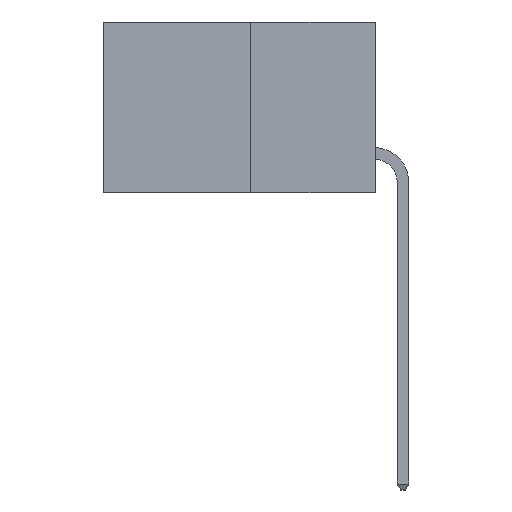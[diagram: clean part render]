
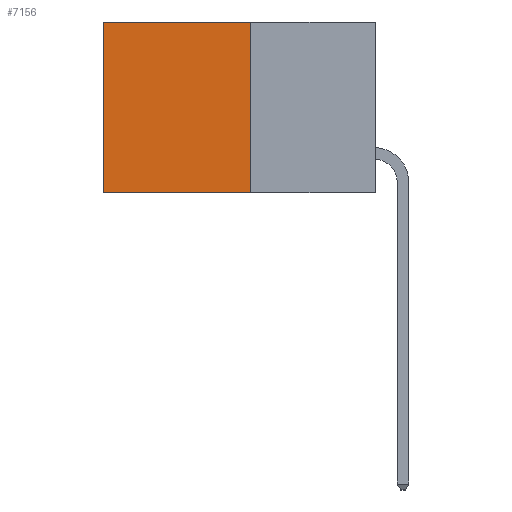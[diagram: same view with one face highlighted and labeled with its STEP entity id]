
A CAD part, left-side view. The second image highlights one B-rep face of the part: STEP entity #7156.
In plain terms, the highlighted planar face has unit normal (-1, 0, 0).
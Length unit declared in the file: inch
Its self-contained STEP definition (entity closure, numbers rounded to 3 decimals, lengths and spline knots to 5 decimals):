
#215 = DIRECTION ( 'NONE',  ( 0., 0., -1. ) ) ;
#286 = VECTOR ( 'NONE', #12590, 39.37008 ) ;
#1157 = LINE ( 'NONE', #21120, #5554 ) ;
#1244 = VERTEX_POINT ( 'NONE', #11138 ) ;
#1817 = VERTEX_POINT ( 'NONE', #10979 ) ;
#2036 = CARTESIAN_POINT ( 'NONE',  ( 0.277, 0.27, -0.37 ) ) ;
#4445 = EDGE_LOOP ( 'NONE', ( #8403, #10588, #11125, #9795 ) ) ;
#5295 = LINE ( 'NONE', #19373, #286 ) ;
#5554 = VECTOR ( 'NONE', #7475, 39.37008 ) ;
#6363 = CARTESIAN_POINT ( 'NONE',  ( 0.277, 0.27, 0. ) ) ;
#7156 = ADVANCED_FACE ( 'NONE', ( #19380 ), #21314, .F. ) ;
#7475 = DIRECTION ( 'NONE',  ( 0., 0., -1. ) ) ;
#7634 = VERTEX_POINT ( 'NONE', #14183 ) ;
#7726 = CARTESIAN_POINT ( 'NONE',  ( 0.277, 0.27, -0.37 ) ) ;
#8145 = DIRECTION ( 'NONE',  ( 0., 1., 0. ) ) ;
#8393 = EDGE_CURVE ( 'NONE', #1817, #7634, #5295, .T. ) ;
#8403 = ORIENTED_EDGE ( 'NONE', *, *, #8393, .T. ) ;
#9428 = VECTOR ( 'NONE', #8145, 39.37008 ) ;
#9455 = DIRECTION ( 'NONE',  ( 0., 1., 0. ) ) ;
#9753 = VERTEX_POINT ( 'NONE', #16592 ) ;
#9770 = AXIS2_PLACEMENT_3D ( 'NONE', #2036, #11075, #215 ) ;
#9795 = ORIENTED_EDGE ( 'NONE', *, *, #12053, .T. ) ;
#10154 = VECTOR ( 'NONE', #9455, 39.37008 ) ;
#10588 = ORIENTED_EDGE ( 'NONE', *, *, #13650, .F. ) ;
#10715 = LINE ( 'NONE', #7726, #10154 ) ;
#10979 = CARTESIAN_POINT ( 'NONE',  ( 0.277, 0.59, 0. ) ) ;
#11075 = DIRECTION ( 'NONE',  ( 1., 0., 0. ) ) ;
#11125 = ORIENTED_EDGE ( 'NONE', *, *, #11747, .F. ) ;
#11138 = CARTESIAN_POINT ( 'NONE',  ( 0.277, 0.27, -0.37 ) ) ;
#11747 = EDGE_CURVE ( 'NONE', #9753, #1244, #1157, .T. ) ;
#12053 = EDGE_CURVE ( 'NONE', #9753, #1817, #19010, .T. ) ;
#12590 = DIRECTION ( 'NONE',  ( 0., 0., -1. ) ) ;
#13650 = EDGE_CURVE ( 'NONE', #1244, #7634, #10715, .T. ) ;
#14183 = CARTESIAN_POINT ( 'NONE',  ( 0.277, 0.59, -0.37 ) ) ;
#16592 = CARTESIAN_POINT ( 'NONE',  ( 0.277, 0.27, 0. ) ) ;
#19010 = LINE ( 'NONE', #6363, #9428 ) ;
#19373 = CARTESIAN_POINT ( 'NONE',  ( 0.277, 0.59, -0.37 ) ) ;
#19380 = FACE_OUTER_BOUND ( 'NONE', #4445, .T. ) ;
#21120 = CARTESIAN_POINT ( 'NONE',  ( 0.277, 0.27, -0.37 ) ) ;
#21314 = PLANE ( 'NONE',  #9770 ) ;
